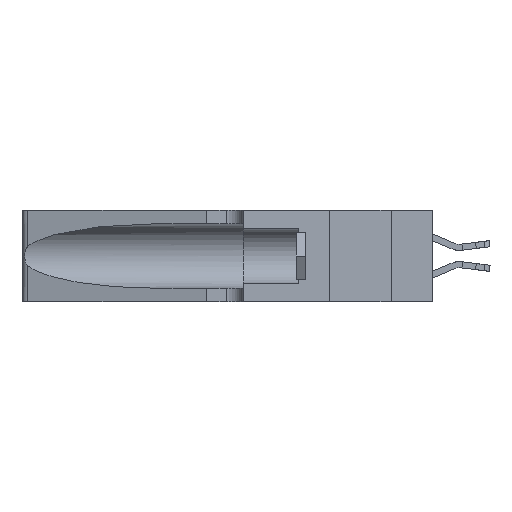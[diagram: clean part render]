
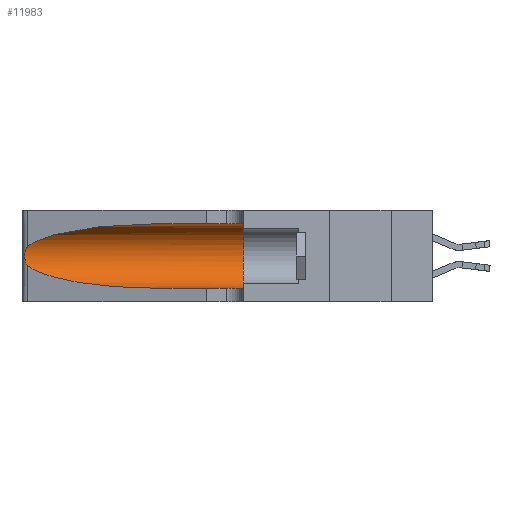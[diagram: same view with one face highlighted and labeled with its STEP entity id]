
A CAD part, left-side view. The second image highlights one B-rep face of the part: STEP entity #11983.
In plain terms, the highlighted cylindrical face has radius 3.308 mm (diameter 6.617 mm), a partial arc.
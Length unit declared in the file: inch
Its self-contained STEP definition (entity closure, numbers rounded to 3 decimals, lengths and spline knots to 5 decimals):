
#11 = CARTESIAN_POINT ( 'NONE',  ( 0.26075, 1.23896, 0.19203 ) ) ;
#273 = CARTESIAN_POINT ( 'NONE',  ( 0.1305, 0.72297, 0.05475 ) ) ;
#347 = ORIENTED_EDGE ( 'NONE', *, *, #10038, .F. ) ;
#398 = CARTESIAN_POINT ( 'NONE',  ( 0.2373, 1.15595, 0.28018 ) ) ;
#912 = ORIENTED_EDGE ( 'NONE', *, *, #14537, .F. ) ;
#1058 =( BOUNDED_CURVE ( )  B_SPLINE_CURVE ( 3, ( #9161, #19506, #398, #12676 ),
 .UNSPECIFIED., .F., .F. ) 
 B_SPLINE_CURVE_WITH_KNOTS ( ( 4, 4 ),
 ( 1.5708, 2.84003 ),
 .UNSPECIFIED. ) 
 CURVE ( )  GEOMETRIC_REPRESENTATION_ITEM ( )  RATIONAL_B_SPLINE_CURVE ( ( 1., 0.87, 0.87, 1. ) ) 
 REPRESENTATION_ITEM ( '' )  );
#1559 = CARTESIAN_POINT ( 'NONE',  ( 0.1305, 0.35, 0.185 ) ) ;
#1579 = CARTESIAN_POINT ( 'NONE',  ( 0.1305, 1.61858, 0.185 ) ) ;
#1866 = CARTESIAN_POINT ( 'NONE',  ( 0.26017, 1.23833, 0.17102 ) ) ;
#1966 = EDGE_LOOP ( 'NONE', ( #22425, #3135, #9118, #15615, #347, #912 ) ) ;
#2064 = VERTEX_POINT ( 'NONE', #21090 ) ;
#2410 =( BOUNDED_CURVE ( )  B_SPLINE_CURVE ( 3, ( #10824, #19387, #7321, #273 ),
 .UNSPECIFIED., .F., .F. ) 
 B_SPLINE_CURVE_WITH_KNOTS ( ( 4, 4 ),
 ( 3.44316, 4.71239 ),
 .UNSPECIFIED. ) 
 CURVE ( )  GEOMETRIC_REPRESENTATION_ITEM ( )  RATIONAL_B_SPLINE_CURVE ( ( 1., 0.87, 0.87, 1. ) ) 
 REPRESENTATION_ITEM ( '' )  );
#3135 = ORIENTED_EDGE ( 'NONE', *, *, #19136, .T. ) ;
#3269 = CARTESIAN_POINT ( 'NONE',  ( 0.1305, 0.35, 0.31525 ) ) ;
#3345 = DIRECTION ( 'NONE',  ( 0., 0., 1. ) ) ;
#3647 = CARTESIAN_POINT ( 'NONE',  ( 0.25789, 1.23486, 0.15765 ) ) ;
#3709 = EDGE_CURVE ( 'NONE', #14165, #8456, #18024, .T. ) ;
#3725 = CARTESIAN_POINT ( 'NONE',  ( 0.1305, 1.61858, 0.05475 ) ) ;
#4218 = CARTESIAN_POINT ( 'NONE',  ( 0.1305, 0.72297, 0.05475 ) ) ;
#4360 = EDGE_CURVE ( 'NONE', #8034, #14165, #2410, .T. ) ;
#5346 = CARTESIAN_POINT ( 'NONE',  ( 0.25555, 1.22994, 0.2215 ) ) ;
#5423 = CARTESIAN_POINT ( 'NONE',  ( 0.25555, 1.22993, 0.14849 ) ) ;
#7321 = CARTESIAN_POINT ( 'NONE',  ( 0.18966, 0.96281, 0.05475 ) ) ;
#8034 = VERTEX_POINT ( 'NONE', #13578 ) ;
#8456 = VERTEX_POINT ( 'NONE', #18056 ) ;
#8744 = CARTESIAN_POINT ( 'NONE',  ( 0.25487, 1.22718, 0.22369 ) ) ;
#8820 = CARTESIAN_POINT ( 'NONE',  ( 0.25787, 1.23484, 0.2124 ) ) ;
#9002 = EDGE_CURVE ( 'NONE', #2064, #18284, #1058, .T. ) ;
#9118 = ORIENTED_EDGE ( 'NONE', *, *, #4360, .T. ) ;
#9161 = CARTESIAN_POINT ( 'NONE',  ( 0.1305, 0.72297, 0.31525 ) ) ;
#10038 = EDGE_CURVE ( 'NONE', #19001, #8456, #22284, .T. ) ;
#10366 = CARTESIAN_POINT ( 'NONE',  ( 0.1305, 1.61858, 0.31525 ) ) ;
#10577 = CARTESIAN_POINT ( 'NONE',  ( 0.26018, 1.23835, 0.19895 ) ) ;
#10824 = CARTESIAN_POINT ( 'NONE',  ( 0.25487, 1.22718, 0.14631 ) ) ;
#11452 = CYLINDRICAL_SURFACE ( 'NONE', #16576, 0.13025 ) ;
#11981 = FACE_OUTER_BOUND ( 'NONE', #1966, .T. ) ;
#11983 = ADVANCED_FACE ( 'NONE', ( #11981 ), #11452, .F. ) ;
#12100 = DIRECTION ( 'NONE',  ( 0., -1., 0. ) ) ;
#12332 = CARTESIAN_POINT ( 'NONE',  ( 0.26075, 1.23896, 0.178 ) ) ;
#12676 = CARTESIAN_POINT ( 'NONE',  ( 0.25487, 1.22718, 0.22369 ) ) ;
#13479 = VECTOR ( 'NONE', #17554, 39.37008 ) ;
#13485 = VECTOR ( 'NONE', #12100, 39.37008 ) ;
#13578 = CARTESIAN_POINT ( 'NONE',  ( 0.25487, 1.22718, 0.14631 ) ) ;
#13759 = DIRECTION ( 'NONE',  ( 0., 1., 0. ) ) ;
#14055 = CARTESIAN_POINT ( 'NONE',  ( 0.25856, 1.23593, 0.16098 ) ) ;
#14165 = VERTEX_POINT ( 'NONE', #4218 ) ;
#14537 = EDGE_CURVE ( 'NONE', #2064, #19001, #18034, .T. ) ;
#14740 = B_SPLINE_CURVE_WITH_KNOTS ( 'NONE', 3,
 ( #8744, #5346, #19153, #8820, #20889, #10577, #11, #12332, #1866, #14055, #3647, #15764, #5423, #17487 ),
 .UNSPECIFIED., .F., .F.,
 ( 4, 2, 2, 2, 2, 2, 4 ),
 ( 0., 0.00027, 0.00053, 0.00107, 0.0016, 0.00187, 0.00214 ),
 .UNSPECIFIED. ) ;
#15615 = ORIENTED_EDGE ( 'NONE', *, *, #3709, .T. ) ;
#15764 = CARTESIAN_POINT ( 'NONE',  ( 0.25639, 1.23186, 0.15144 ) ) ;
#16576 = AXIS2_PLACEMENT_3D ( 'NONE', #1579, #22375, #17133 ) ;
#17133 = DIRECTION ( 'NONE',  ( 0., 0., -1. ) ) ;
#17487 = CARTESIAN_POINT ( 'NONE',  ( 0.25487, 1.22718, 0.14631 ) ) ;
#17554 = DIRECTION ( 'NONE',  ( 0., -1., 0. ) ) ;
#17988 = AXIS2_PLACEMENT_3D ( 'NONE', #1559, #13759, #3345 ) ;
#18024 = LINE ( 'NONE', #3725, #13479 ) ;
#18034 = LINE ( 'NONE', #10366, #13485 ) ;
#18056 = CARTESIAN_POINT ( 'NONE',  ( 0.1305, 0.35, 0.05475 ) ) ;
#18284 = VERTEX_POINT ( 'NONE', #18739 ) ;
#18739 = CARTESIAN_POINT ( 'NONE',  ( 0.25487, 1.22718, 0.22369 ) ) ;
#19001 = VERTEX_POINT ( 'NONE', #3269 ) ;
#19136 = EDGE_CURVE ( 'NONE', #18284, #8034, #14740, .T. ) ;
#19153 = CARTESIAN_POINT ( 'NONE',  ( 0.25639, 1.23184, 0.21858 ) ) ;
#19387 = CARTESIAN_POINT ( 'NONE',  ( 0.2373, 1.15595, 0.08982 ) ) ;
#19506 = CARTESIAN_POINT ( 'NONE',  ( 0.18966, 0.96281, 0.31525 ) ) ;
#20889 = CARTESIAN_POINT ( 'NONE',  ( 0.25854, 1.2359, 0.20912 ) ) ;
#21090 = CARTESIAN_POINT ( 'NONE',  ( 0.1305, 0.72297, 0.31525 ) ) ;
#22284 = CIRCLE ( 'NONE', #17988, 0.13025 ) ;
#22375 = DIRECTION ( 'NONE',  ( 0., -1., 0. ) ) ;
#22425 = ORIENTED_EDGE ( 'NONE', *, *, #9002, .T. ) ;
